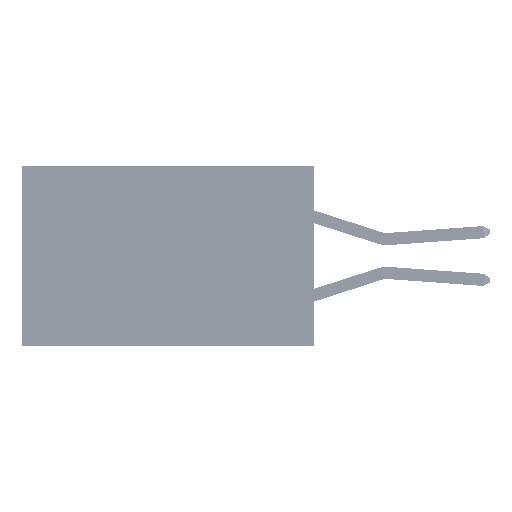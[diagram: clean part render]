
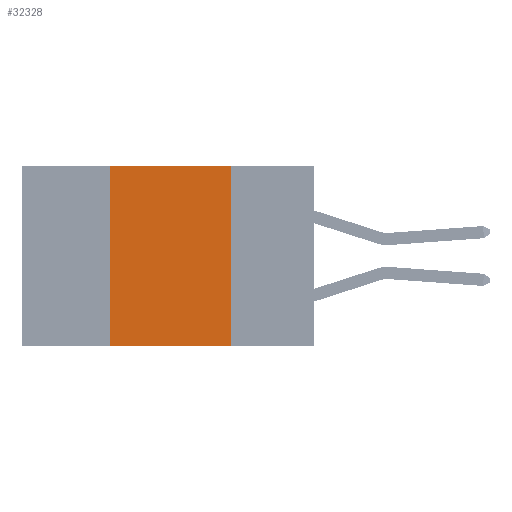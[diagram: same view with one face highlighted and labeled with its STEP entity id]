
A CAD part, left-side view. The second image highlights one B-rep face of the part: STEP entity #32328.
In plain terms, the highlighted planar face has unit normal (-1, 0, 0).
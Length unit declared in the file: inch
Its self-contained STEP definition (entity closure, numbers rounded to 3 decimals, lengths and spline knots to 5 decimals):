
#1576 = VERTEX_POINT ( 'NONE', #11132 ) ;
#2065 = DIRECTION ( 'NONE',  ( 0., 0., -1. ) ) ;
#2891 = AXIS2_PLACEMENT_3D ( 'NONE', #9564, #20563, #25139 ) ;
#2966 = VECTOR ( 'NONE', #2065, 39.37008 ) ;
#5720 = DIRECTION ( 'NONE',  ( 0., -1., 0. ) ) ;
#7387 = VERTEX_POINT ( 'NONE', #39352 ) ;
#8578 = VERTEX_POINT ( 'NONE', #29740 ) ;
#9564 = CARTESIAN_POINT ( 'NONE',  ( 0., 0.6, 0. ) ) ;
#11132 = CARTESIAN_POINT ( 'NONE',  ( 0., 0.17, 0. ) ) ;
#11327 = ORIENTED_EDGE ( 'NONE', *, *, #41109, .F. ) ;
#16721 = PLANE ( 'NONE',  #2891 ) ;
#17787 = EDGE_CURVE ( 'NONE', #1576, #8578, #25321, .T. ) ;
#18543 = LINE ( 'NONE', #26208, #49030 ) ;
#20563 = DIRECTION ( 'NONE',  ( 1., 0., 0. ) ) ;
#21755 = EDGE_CURVE ( 'NONE', #7387, #8578, #36915, .T. ) ;
#23034 = VECTOR ( 'NONE', #5720, 39.37008 ) ;
#25139 = DIRECTION ( 'NONE',  ( 0., 0., -1. ) ) ;
#25321 = LINE ( 'NONE', #37104, #2966 ) ;
#26208 = CARTESIAN_POINT ( 'NONE',  ( 0., 0.42, 0. ) ) ;
#28003 = EDGE_CURVE ( 'NONE', #7387, #31902, #18543, .T. ) ;
#29740 = CARTESIAN_POINT ( 'NONE',  ( 0., 0.17, -0.37 ) ) ;
#29823 = ORIENTED_EDGE ( 'NONE', *, *, #17787, .F. ) ;
#31730 = CARTESIAN_POINT ( 'NONE',  ( 0., 0.42, 0. ) ) ;
#31902 = VERTEX_POINT ( 'NONE', #31730 ) ;
#31955 = ORIENTED_EDGE ( 'NONE', *, *, #21755, .T. ) ;
#32328 = ADVANCED_FACE ( 'NONE', ( #36924 ), #16721, .F. ) ;
#33592 = CARTESIAN_POINT ( 'NONE',  ( 0., 0.6, -0.37 ) ) ;
#33701 = EDGE_LOOP ( 'NONE', ( #29823, #11327, #47581, #31955 ) ) ;
#36915 = LINE ( 'NONE', #33592, #23034 ) ;
#36924 = FACE_OUTER_BOUND ( 'NONE', #33701, .T. ) ;
#37104 = CARTESIAN_POINT ( 'NONE',  ( 0., 0.17, 0. ) ) ;
#37486 = DIRECTION ( 'NONE',  ( 0., 0., 1. ) ) ;
#39352 = CARTESIAN_POINT ( 'NONE',  ( 0., 0.42, -0.37 ) ) ;
#39766 = VECTOR ( 'NONE', #40987, 39.37008 ) ;
#40735 = CARTESIAN_POINT ( 'NONE',  ( 0., 0.6, 0. ) ) ;
#40987 = DIRECTION ( 'NONE',  ( 0., -1., 0. ) ) ;
#41109 = EDGE_CURVE ( 'NONE', #31902, #1576, #49182, .T. ) ;
#47581 = ORIENTED_EDGE ( 'NONE', *, *, #28003, .F. ) ;
#49030 = VECTOR ( 'NONE', #37486, 39.37008 ) ;
#49182 = LINE ( 'NONE', #40735, #39766 ) ;
